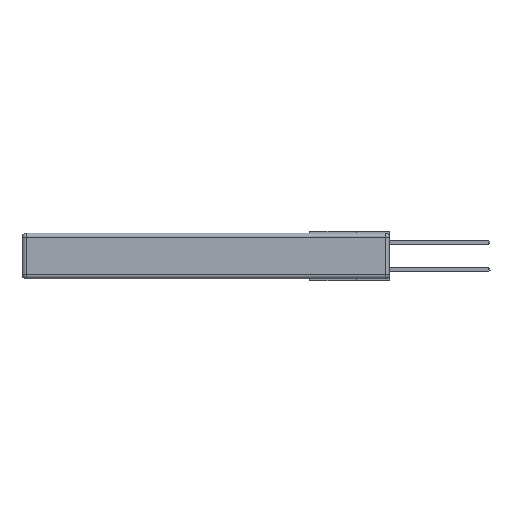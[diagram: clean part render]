
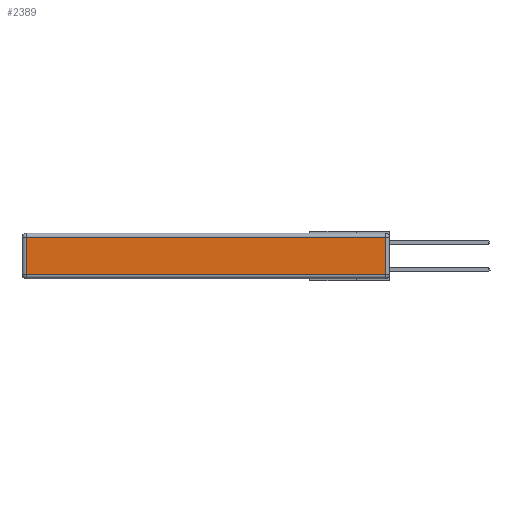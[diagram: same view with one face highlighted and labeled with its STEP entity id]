
A CAD part, left-side view. The second image highlights one B-rep face of the part: STEP entity #2389.
In plain terms, the highlighted planar face has unit normal (-1, 0, 0).
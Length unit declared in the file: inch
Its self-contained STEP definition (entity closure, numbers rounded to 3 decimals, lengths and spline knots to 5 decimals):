
#1299 = AXIS2_PLACEMENT_3D ( 'NONE', #9752, #11792, #3360 ) ;
#1462 = EDGE_CURVE ( 'NONE', #12876, #10431, #7534, .T. ) ;
#2389 = ADVANCED_FACE ( 'NONE', ( #11029 ), #4390, .T. ) ;
#2849 = CARTESIAN_POINT ( 'NONE',  ( 0., 2.72, -0.343 ) ) ;
#2888 = DIRECTION ( 'NONE',  ( 0., 0., -1. ) ) ;
#3025 = EDGE_CURVE ( 'NONE', #10431, #13397, #12651, .T. ) ;
#3204 = CARTESIAN_POINT ( 'NONE',  ( 0., 2.72, -0.313 ) ) ;
#3360 = DIRECTION ( 'NONE',  ( 0., 0., 1. ) ) ;
#3713 = CARTESIAN_POINT ( 'NONE',  ( 0., 0.03, -0.343 ) ) ;
#4141 = ORIENTED_EDGE ( 'NONE', *, *, #1462, .T. ) ;
#4207 = ORIENTED_EDGE ( 'NONE', *, *, #10697, .T. ) ;
#4390 = PLANE ( 'NONE',  #1299 ) ;
#4819 = CARTESIAN_POINT ( 'NONE',  ( 0., 0.03, -0.03 ) ) ;
#5028 = VECTOR ( 'NONE', #8789, 39.37008 ) ;
#5251 = ORIENTED_EDGE ( 'NONE', *, *, #3025, .T. ) ;
#6038 = DIRECTION ( 'NONE',  ( 0., 1., 0. ) ) ;
#6208 = LINE ( 'NONE', #11837, #5028 ) ;
#7534 = LINE ( 'NONE', #3713, #12846 ) ;
#8655 = VECTOR ( 'NONE', #2888, 39.37008 ) ;
#8789 = DIRECTION ( 'NONE',  ( 0., -1., 0. ) ) ;
#9347 = EDGE_LOOP ( 'NONE', ( #4207, #4141, #5251, #13494 ) ) ;
#9752 = CARTESIAN_POINT ( 'NONE',  ( 0., 0., -0.343 ) ) ;
#9837 = VERTEX_POINT ( 'NONE', #3204 ) ;
#10335 = CARTESIAN_POINT ( 'NONE',  ( 0., 2.72, -0.03 ) ) ;
#10431 = VERTEX_POINT ( 'NONE', #4819 ) ;
#10697 = EDGE_CURVE ( 'NONE', #9837, #12876, #6208, .T. ) ;
#11029 = FACE_OUTER_BOUND ( 'NONE', #9347, .T. ) ;
#11146 = LINE ( 'NONE', #2849, #8655 ) ;
#11167 = VECTOR ( 'NONE', #6038, 39.37008 ) ;
#11792 = DIRECTION ( 'NONE',  ( -1., 0., 0. ) ) ;
#11837 = CARTESIAN_POINT ( 'NONE',  ( 0., 0., -0.313 ) ) ;
#12153 = DIRECTION ( 'NONE',  ( 0., 0., 1. ) ) ;
#12401 = CARTESIAN_POINT ( 'NONE',  ( 0., 2.75, -0.03 ) ) ;
#12651 = LINE ( 'NONE', #12401, #11167 ) ;
#12674 = EDGE_CURVE ( 'NONE', #13397, #9837, #11146, .T. ) ;
#12846 = VECTOR ( 'NONE', #12153, 39.37008 ) ;
#12876 = VERTEX_POINT ( 'NONE', #12890 ) ;
#12890 = CARTESIAN_POINT ( 'NONE',  ( 0., 0.03, -0.313 ) ) ;
#13397 = VERTEX_POINT ( 'NONE', #10335 ) ;
#13494 = ORIENTED_EDGE ( 'NONE', *, *, #12674, .T. ) ;
